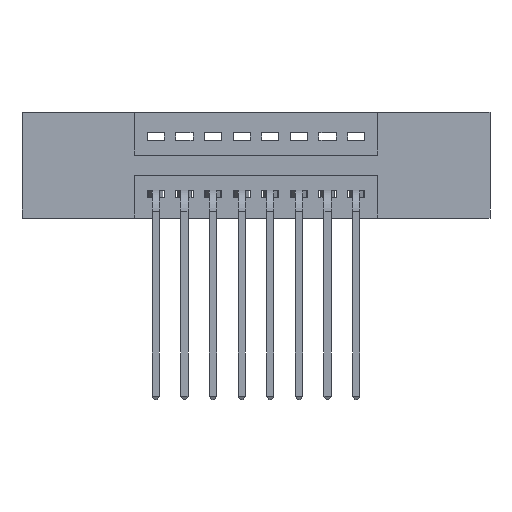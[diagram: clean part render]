
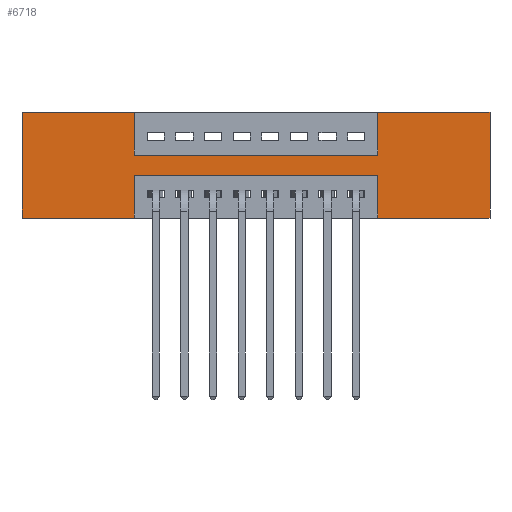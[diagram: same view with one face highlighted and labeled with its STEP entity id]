
A CAD part, front view. The second image highlights one B-rep face of the part: STEP entity #6718.
In plain terms, the highlighted planar face has unit normal (0, -1, 0).
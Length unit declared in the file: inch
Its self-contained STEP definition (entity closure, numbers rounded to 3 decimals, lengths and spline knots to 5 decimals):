
#57 = ORIENTED_EDGE ( 'NONE', *, *, #4731, .F. ) ;
#59 = VERTEX_POINT ( 'NONE', #4606 ) ;
#140 = CARTESIAN_POINT ( 'NONE',  ( 1.635, 0., 0. ) ) ;
#179 = ORIENTED_EDGE ( 'NONE', *, *, #8021, .F. ) ;
#276 = CARTESIAN_POINT ( 'NONE',  ( 1.2425, 0., -0.37 ) ) ;
#307 = EDGE_CURVE ( 'NONE', #927, #9102, #2315, .T. ) ;
#548 = CARTESIAN_POINT ( 'NONE',  ( 1.2425, 0., -0.15 ) ) ;
#578 = VECTOR ( 'NONE', #1176, 39.37008 ) ;
#594 = PLANE ( 'NONE',  #5025 ) ;
#775 = CARTESIAN_POINT ( 'NONE',  ( 1.635, 0., -0.37 ) ) ;
#891 = VERTEX_POINT ( 'NONE', #5015 ) ;
#927 = VERTEX_POINT ( 'NONE', #5221 ) ;
#962 = DIRECTION ( 'NONE',  ( 0., 0., 1. ) ) ;
#1176 = DIRECTION ( 'NONE',  ( -1., 0., 0. ) ) ;
#1204 = VECTOR ( 'NONE', #10700, 39.37008 ) ;
#1443 = VECTOR ( 'NONE', #9945, 39.37008 ) ;
#1500 = LINE ( 'NONE', #6552, #4445 ) ;
#1734 = VECTOR ( 'NONE', #3909, 39.37008 ) ;
#1742 = DIRECTION ( 'NONE',  ( 0., 0., -1. ) ) ;
#1815 = VERTEX_POINT ( 'NONE', #548 ) ;
#1968 = VERTEX_POINT ( 'NONE', #4067 ) ;
#1978 = CARTESIAN_POINT ( 'NONE',  ( 0.3925, 0., -0.15 ) ) ;
#2012 = LINE ( 'NONE', #5888, #10520 ) ;
#2021 = ORIENTED_EDGE ( 'NONE', *, *, #7293, .F. ) ;
#2085 = VECTOR ( 'NONE', #962, 39.37008 ) ;
#2177 = EDGE_CURVE ( 'NONE', #7653, #891, #9015, .T. ) ;
#2315 = LINE ( 'NONE', #8656, #6131 ) ;
#2630 = LINE ( 'NONE', #3612, #578 ) ;
#2716 = DIRECTION ( 'NONE',  ( 0., 0., 1. ) ) ;
#2842 = DIRECTION ( 'NONE',  ( 0., 0., -1. ) ) ;
#2890 = VERTEX_POINT ( 'NONE', #1978 ) ;
#2898 = DIRECTION ( 'NONE',  ( -1., 0., 0. ) ) ;
#3107 = CARTESIAN_POINT ( 'NONE',  ( 0., 0., 0. ) ) ;
#3612 = CARTESIAN_POINT ( 'NONE',  ( 0., 0., -0.37 ) ) ;
#3909 = DIRECTION ( 'NONE',  ( 1., 0., 0. ) ) ;
#4067 = CARTESIAN_POINT ( 'NONE',  ( 0., 0., 0. ) ) ;
#4157 = VERTEX_POINT ( 'NONE', #6090 ) ;
#4249 = LINE ( 'NONE', #276, #10599 ) ;
#4254 = VECTOR ( 'NONE', #9095, 39.37008 ) ;
#4445 = VECTOR ( 'NONE', #1742, 39.37008 ) ;
#4606 = CARTESIAN_POINT ( 'NONE',  ( 1.2425, 0., 0. ) ) ;
#4645 = FACE_OUTER_BOUND ( 'NONE', #5702, .T. ) ;
#4731 = EDGE_CURVE ( 'NONE', #4157, #2890, #1500, .T. ) ;
#4753 = VERTEX_POINT ( 'NONE', #8190 ) ;
#4875 = CARTESIAN_POINT ( 'NONE',  ( 0.3925, 0., -0.22 ) ) ;
#4886 = CARTESIAN_POINT ( 'NONE',  ( 0.3925, 0., -0.37 ) ) ;
#4970 = DIRECTION ( 'NONE',  ( 0., 0., 1. ) ) ;
#5015 = CARTESIAN_POINT ( 'NONE',  ( 0., 0., -0.37 ) ) ;
#5025 = AXIS2_PLACEMENT_3D ( 'NONE', #7093, #8802, #8653 ) ;
#5171 = EDGE_CURVE ( 'NONE', #891, #1968, #2012, .T. ) ;
#5221 = CARTESIAN_POINT ( 'NONE',  ( 1.2425, 0., -0.22 ) ) ;
#5252 = ORIENTED_EDGE ( 'NONE', *, *, #5171, .F. ) ;
#5304 = ORIENTED_EDGE ( 'NONE', *, *, #5947, .F. ) ;
#5331 = CARTESIAN_POINT ( 'NONE',  ( 1.635, 0., 0. ) ) ;
#5382 = EDGE_CURVE ( 'NONE', #9102, #7653, #6720, .T. ) ;
#5581 = ORIENTED_EDGE ( 'NONE', *, *, #9440, .F. ) ;
#5702 = EDGE_LOOP ( 'NONE', ( #9689, #10560, #5581, #9659, #5304, #7617, #2021, #6004, #57, #179, #5252, #8144 ) ) ;
#5887 = VECTOR ( 'NONE', #2898, 39.37008 ) ;
#5888 = CARTESIAN_POINT ( 'NONE',  ( 0., 0., 0. ) ) ;
#5947 = EDGE_CURVE ( 'NONE', #9602, #8103, #6064, .T. ) ;
#6004 = ORIENTED_EDGE ( 'NONE', *, *, #7167, .F. ) ;
#6042 = DIRECTION ( 'NONE',  ( -1., 0., 0. ) ) ;
#6064 = LINE ( 'NONE', #140, #1204 ) ;
#6090 = CARTESIAN_POINT ( 'NONE',  ( 0.3925, 0., 0. ) ) ;
#6125 = EDGE_CURVE ( 'NONE', #8103, #4753, #2630, .T. ) ;
#6131 = VECTOR ( 'NONE', #6042, 39.37008 ) ;
#6552 = CARTESIAN_POINT ( 'NONE',  ( 0.3925, 0., 0. ) ) ;
#6718 = ADVANCED_FACE ( 'NONE', ( #4645 ), #594, .T. ) ;
#6720 = LINE ( 'NONE', #10569, #8181 ) ;
#6941 = LINE ( 'NONE', #8505, #2085 ) ;
#7093 = CARTESIAN_POINT ( 'NONE',  ( 0., 0., -0.37 ) ) ;
#7163 = EDGE_CURVE ( 'NONE', #59, #9602, #10602, .T. ) ;
#7167 = EDGE_CURVE ( 'NONE', #2890, #1815, #7487, .T. ) ;
#7293 = EDGE_CURVE ( 'NONE', #1815, #59, #6941, .T. ) ;
#7487 = LINE ( 'NONE', #7801, #1443 ) ;
#7617 = ORIENTED_EDGE ( 'NONE', *, *, #7163, .F. ) ;
#7653 = VERTEX_POINT ( 'NONE', #4886 ) ;
#7801 = CARTESIAN_POINT ( 'NONE',  ( 0.3925, 0., -0.15 ) ) ;
#8021 = EDGE_CURVE ( 'NONE', #1968, #4157, #8294, .T. ) ;
#8103 = VERTEX_POINT ( 'NONE', #775 ) ;
#8144 = ORIENTED_EDGE ( 'NONE', *, *, #2177, .F. ) ;
#8181 = VECTOR ( 'NONE', #2842, 39.37008 ) ;
#8190 = CARTESIAN_POINT ( 'NONE',  ( 1.2425, 0., -0.37 ) ) ;
#8294 = LINE ( 'NONE', #3107, #1734 ) ;
#8505 = CARTESIAN_POINT ( 'NONE',  ( 1.2425, 0., 0. ) ) ;
#8653 = DIRECTION ( 'NONE',  ( 0., 0., -1. ) ) ;
#8656 = CARTESIAN_POINT ( 'NONE',  ( 0.3925, 0., -0.22 ) ) ;
#8802 = DIRECTION ( 'NONE',  ( 0., -1., 0. ) ) ;
#9015 = LINE ( 'NONE', #9430, #5887 ) ;
#9095 = DIRECTION ( 'NONE',  ( 1., 0., 0. ) ) ;
#9102 = VERTEX_POINT ( 'NONE', #4875 ) ;
#9430 = CARTESIAN_POINT ( 'NONE',  ( 0., 0., -0.37 ) ) ;
#9440 = EDGE_CURVE ( 'NONE', #4753, #927, #4249, .T. ) ;
#9602 = VERTEX_POINT ( 'NONE', #5331 ) ;
#9659 = ORIENTED_EDGE ( 'NONE', *, *, #6125, .F. ) ;
#9689 = ORIENTED_EDGE ( 'NONE', *, *, #5382, .F. ) ;
#9945 = DIRECTION ( 'NONE',  ( 1., 0., 0. ) ) ;
#10027 = CARTESIAN_POINT ( 'NONE',  ( 0., 0., 0. ) ) ;
#10520 = VECTOR ( 'NONE', #4970, 39.37008 ) ;
#10560 = ORIENTED_EDGE ( 'NONE', *, *, #307, .F. ) ;
#10569 = CARTESIAN_POINT ( 'NONE',  ( 0.3925, 0., -0.37 ) ) ;
#10599 = VECTOR ( 'NONE', #2716, 39.37008 ) ;
#10602 = LINE ( 'NONE', #10027, #4254 ) ;
#10700 = DIRECTION ( 'NONE',  ( 0., 0., -1. ) ) ;
